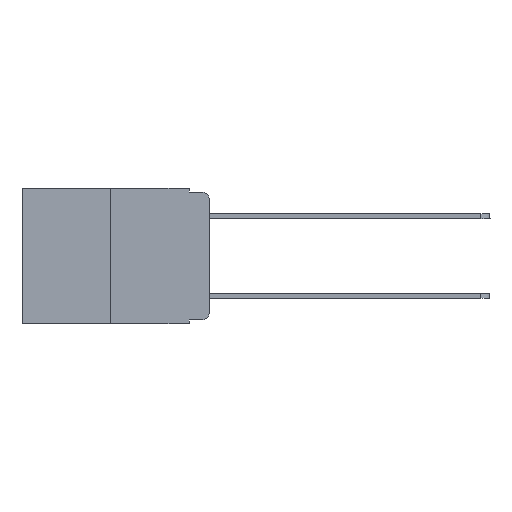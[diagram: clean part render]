
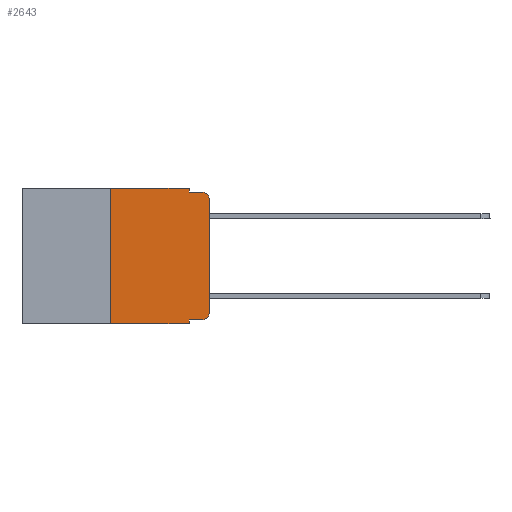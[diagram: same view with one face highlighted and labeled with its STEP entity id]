
A CAD part, left-side view. The second image highlights one B-rep face of the part: STEP entity #2643.
In plain terms, the highlighted planar face has unit normal (-1, 0, 0).
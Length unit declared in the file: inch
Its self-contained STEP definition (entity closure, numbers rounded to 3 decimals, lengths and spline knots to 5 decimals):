
#105 = DIRECTION ( 'NONE',  ( 0., -1., 0. ) ) ;
#288 = LINE ( 'NONE', #12283, #4777 ) ;
#454 = LINE ( 'NONE', #4728, #5543 ) ;
#458 = ORIENTED_EDGE ( 'NONE', *, *, #4875, .T. ) ;
#519 = EDGE_CURVE ( 'NONE', #5767, #7605, #10136, .T. ) ;
#958 = CARTESIAN_POINT ( 'NONE',  ( 0., 0.25, 0. ) ) ;
#1252 = EDGE_CURVE ( 'NONE', #2134, #4017, #13055, .T. ) ;
#1328 = EDGE_CURVE ( 'NONE', #3929, #12610, #9955, .T. ) ;
#1511 = VECTOR ( 'NONE', #10056, 39.37008 ) ;
#1749 = CARTESIAN_POINT ( 'NONE',  ( 0., 0., -0.313 ) ) ;
#1835 = EDGE_LOOP ( 'NONE', ( #9104, #3191, #4335, #4997, #11146, #9464, #458, #7920, #6824, #5032 ) ) ;
#2134 = VERTEX_POINT ( 'NONE', #4609 ) ;
#2285 = DIRECTION ( 'NONE',  ( 0., 0., -1. ) ) ;
#2328 = CARTESIAN_POINT ( 'NONE',  ( 0., 0.25, 0. ) ) ;
#2643 = ADVANCED_FACE ( 'NONE', ( #7898 ), #2867, .F. ) ;
#2867 = PLANE ( 'NONE',  #10523 ) ;
#2879 = LINE ( 'NONE', #6029, #7716 ) ;
#2891 = CARTESIAN_POINT ( 'NONE',  ( 0., 0., 0. ) ) ;
#3191 = ORIENTED_EDGE ( 'NONE', *, *, #1252, .T. ) ;
#3326 = CARTESIAN_POINT ( 'NONE',  ( 0., 0.051, -0.01 ) ) ;
#3451 = DIRECTION ( 'NONE',  ( 0., -1., 0. ) ) ;
#3716 = DIRECTION ( 'NONE',  ( 1., 0., 0. ) ) ;
#3929 = VERTEX_POINT ( 'NONE', #9204 ) ;
#3998 = LINE ( 'NONE', #10185, #1511 ) ;
#4011 = VECTOR ( 'NONE', #5911, 39.37008 ) ;
#4017 = VERTEX_POINT ( 'NONE', #12337 ) ;
#4063 = DIRECTION ( 'NONE',  ( 0., 0., -1. ) ) ;
#4148 = CARTESIAN_POINT ( 'NONE',  ( 0., 0.051, 0. ) ) ;
#4320 = CARTESIAN_POINT ( 'NONE',  ( 0., 0.25, -0.343 ) ) ;
#4335 = ORIENTED_EDGE ( 'NONE', *, *, #7679, .F. ) ;
#4609 = CARTESIAN_POINT ( 'NONE',  ( 0., 0., -0.03 ) ) ;
#4728 = CARTESIAN_POINT ( 'NONE',  ( 0., 0.051, -0.01 ) ) ;
#4730 = DIRECTION ( 'NONE',  ( 0., 0., -1. ) ) ;
#4777 = VECTOR ( 'NONE', #105, 39.37008 ) ;
#4875 = EDGE_CURVE ( 'NONE', #5767, #7539, #288, .T. ) ;
#4997 = ORIENTED_EDGE ( 'NONE', *, *, #10091, .F. ) ;
#5032 = ORIENTED_EDGE ( 'NONE', *, *, #7550, .T. ) ;
#5176 = EDGE_CURVE ( 'NONE', #6751, #2134, #11933, .T. ) ;
#5543 = VECTOR ( 'NONE', #3451, 39.37008 ) ;
#5767 = VERTEX_POINT ( 'NONE', #4320 ) ;
#5911 = DIRECTION ( 'NONE',  ( 0., 0., 1. ) ) ;
#5944 = CARTESIAN_POINT ( 'NONE',  ( 0., 0.473, 0. ) ) ;
#5956 = CARTESIAN_POINT ( 'NONE',  ( 0., 0.02, -0.313 ) ) ;
#6029 = CARTESIAN_POINT ( 'NONE',  ( 0., 0.051, 0. ) ) ;
#6096 = CARTESIAN_POINT ( 'NONE',  ( 0., 0.051, -0.343 ) ) ;
#6751 = VERTEX_POINT ( 'NONE', #1749 ) ;
#6824 = ORIENTED_EDGE ( 'NONE', *, *, #1328, .T. ) ;
#7289 = CIRCLE ( 'NONE', #10466, 0.02 ) ;
#7408 = EDGE_CURVE ( 'NONE', #7605, #12900, #3998, .T. ) ;
#7471 = CARTESIAN_POINT ( 'NONE',  ( 0., 0.02, -0.333 ) ) ;
#7478 = AXIS2_PLACEMENT_3D ( 'NONE', #12717, #7503, #7566 ) ;
#7503 = DIRECTION ( 'NONE',  ( -1., 0., 0. ) ) ;
#7517 = EDGE_CURVE ( 'NONE', #3929, #7539, #2879, .T. ) ;
#7539 = VERTEX_POINT ( 'NONE', #6096 ) ;
#7550 = EDGE_CURVE ( 'NONE', #12610, #6751, #7289, .T. ) ;
#7566 = DIRECTION ( 'NONE',  ( 0., 0., -1. ) ) ;
#7605 = VERTEX_POINT ( 'NONE', #2328 ) ;
#7679 = EDGE_CURVE ( 'NONE', #10725, #4017, #454, .T. ) ;
#7716 = VECTOR ( 'NONE', #4063, 39.37008 ) ;
#7898 = FACE_OUTER_BOUND ( 'NONE', #1835, .T. ) ;
#7916 = DIRECTION ( 'NONE',  ( 0., 0., -1. ) ) ;
#7920 = ORIENTED_EDGE ( 'NONE', *, *, #7517, .F. ) ;
#8873 = DIRECTION ( 'NONE',  ( 0., 0., 1. ) ) ;
#9104 = ORIENTED_EDGE ( 'NONE', *, *, #5176, .T. ) ;
#9204 = CARTESIAN_POINT ( 'NONE',  ( 0., 0.051, -0.333 ) ) ;
#9228 = DIRECTION ( 'NONE',  ( 0., -1., 0. ) ) ;
#9464 = ORIENTED_EDGE ( 'NONE', *, *, #519, .F. ) ;
#9955 = LINE ( 'NONE', #10086, #10898 ) ;
#10056 = DIRECTION ( 'NONE',  ( 0., -1., 0. ) ) ;
#10086 = CARTESIAN_POINT ( 'NONE',  ( 0., 0.051, -0.333 ) ) ;
#10091 = EDGE_CURVE ( 'NONE', #12900, #10725, #11339, .T. ) ;
#10136 = LINE ( 'NONE', #958, #4011 ) ;
#10185 = CARTESIAN_POINT ( 'NONE',  ( 0., 0.473, 0. ) ) ;
#10243 = DIRECTION ( 'NONE',  ( -1., 0., 0. ) ) ;
#10466 = AXIS2_PLACEMENT_3D ( 'NONE', #5956, #10243, #7916 ) ;
#10523 = AXIS2_PLACEMENT_3D ( 'NONE', #5944, #3716, #4730 ) ;
#10534 = VECTOR ( 'NONE', #2285, 39.37008 ) ;
#10725 = VERTEX_POINT ( 'NONE', #3326 ) ;
#10898 = VECTOR ( 'NONE', #9228, 39.37008 ) ;
#11146 = ORIENTED_EDGE ( 'NONE', *, *, #7408, .F. ) ;
#11339 = LINE ( 'NONE', #4148, #10534 ) ;
#11933 = LINE ( 'NONE', #2891, #12836 ) ;
#12283 = CARTESIAN_POINT ( 'NONE',  ( 0., 0.473, -0.343 ) ) ;
#12337 = CARTESIAN_POINT ( 'NONE',  ( 0., 0.02, -0.01 ) ) ;
#12610 = VERTEX_POINT ( 'NONE', #7471 ) ;
#12691 = CARTESIAN_POINT ( 'NONE',  ( 0., 0.051, 0. ) ) ;
#12717 = CARTESIAN_POINT ( 'NONE',  ( 0., 0.02, -0.03 ) ) ;
#12836 = VECTOR ( 'NONE', #8873, 39.37008 ) ;
#12900 = VERTEX_POINT ( 'NONE', #12691 ) ;
#13055 = CIRCLE ( 'NONE', #7478, 0.02 ) ;
